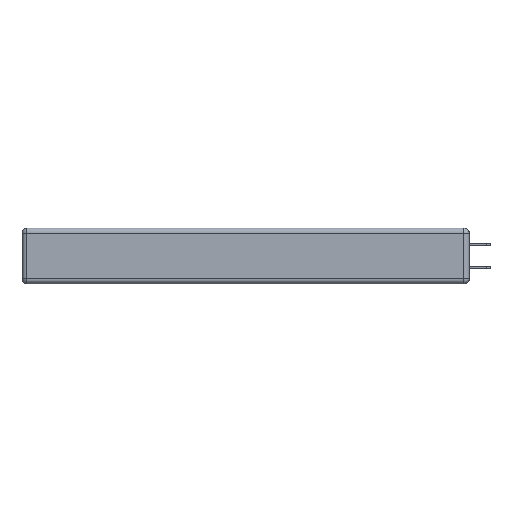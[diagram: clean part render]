
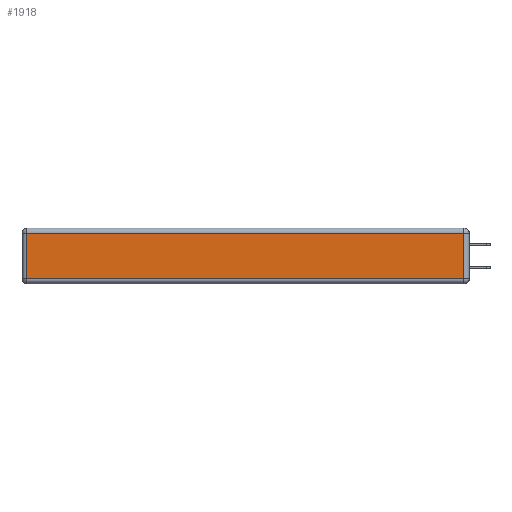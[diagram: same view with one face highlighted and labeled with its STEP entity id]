
A CAD part, left-side view. The second image highlights one B-rep face of the part: STEP entity #1918.
In plain terms, the highlighted planar face has unit normal (-1, 0, 0).
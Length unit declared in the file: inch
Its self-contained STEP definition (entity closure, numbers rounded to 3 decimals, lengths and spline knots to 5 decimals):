
#1327 = VECTOR ( 'NONE', #1982, 39.37008 ) ;
#1918 = ADVANCED_FACE ( 'NONE', ( #12549 ), #13096, .T. ) ;
#1982 = DIRECTION ( 'NONE',  ( 0., 1., 0. ) ) ;
#2371 = LINE ( 'NONE', #9660, #13173 ) ;
#2747 = ORIENTED_EDGE ( 'NONE', *, *, #12904, .T. ) ;
#2912 = AXIS2_PLACEMENT_3D ( 'NONE', #13278, #8189, #12278 ) ;
#3001 = ORIENTED_EDGE ( 'NONE', *, *, #13464, .T. ) ;
#4315 = VERTEX_POINT ( 'NONE', #12604 ) ;
#4664 = EDGE_CURVE ( 'NONE', #5330, #4315, #2371, .T. ) ;
#4808 = LINE ( 'NONE', #6531, #10383 ) ;
#5114 = CARTESIAN_POINT ( 'NONE',  ( 0., 2.72, -0.03 ) ) ;
#5116 = LINE ( 'NONE', #10831, #12792 ) ;
#5330 = VERTEX_POINT ( 'NONE', #13108 ) ;
#6531 = CARTESIAN_POINT ( 'NONE',  ( 0., 0., -0.313 ) ) ;
#7487 = EDGE_CURVE ( 'NONE', #4315, #8409, #12140, .T. ) ;
#8148 = CARTESIAN_POINT ( 'NONE',  ( 0., 2.72, -0.313 ) ) ;
#8189 = DIRECTION ( 'NONE',  ( -1., 0., 0. ) ) ;
#8409 = VERTEX_POINT ( 'NONE', #5114 ) ;
#9660 = CARTESIAN_POINT ( 'NONE',  ( 0., 0.03, -0.343 ) ) ;
#9910 = ORIENTED_EDGE ( 'NONE', *, *, #7487, .T. ) ;
#9973 = ORIENTED_EDGE ( 'NONE', *, *, #4664, .T. ) ;
#10188 = VERTEX_POINT ( 'NONE', #8148 ) ;
#10383 = VECTOR ( 'NONE', #12887, 39.37008 ) ;
#10702 = DIRECTION ( 'NONE',  ( 0., 0., -1. ) ) ;
#10831 = CARTESIAN_POINT ( 'NONE',  ( 0., 2.72, -0.343 ) ) ;
#10891 = EDGE_LOOP ( 'NONE', ( #2747, #9973, #9910, #3001 ) ) ;
#11318 = CARTESIAN_POINT ( 'NONE',  ( 0., 2.75, -0.03 ) ) ;
#12140 = LINE ( 'NONE', #11318, #1327 ) ;
#12278 = DIRECTION ( 'NONE',  ( 0., 0., 1. ) ) ;
#12549 = FACE_OUTER_BOUND ( 'NONE', #10891, .T. ) ;
#12604 = CARTESIAN_POINT ( 'NONE',  ( 0., 0.03, -0.03 ) ) ;
#12772 = DIRECTION ( 'NONE',  ( 0., 0., 1. ) ) ;
#12792 = VECTOR ( 'NONE', #10702, 39.37008 ) ;
#12887 = DIRECTION ( 'NONE',  ( 0., -1., 0. ) ) ;
#12904 = EDGE_CURVE ( 'NONE', #10188, #5330, #4808, .T. ) ;
#13096 = PLANE ( 'NONE',  #2912 ) ;
#13108 = CARTESIAN_POINT ( 'NONE',  ( 0., 0.03, -0.313 ) ) ;
#13173 = VECTOR ( 'NONE', #12772, 39.37008 ) ;
#13278 = CARTESIAN_POINT ( 'NONE',  ( 0., 0., -0.343 ) ) ;
#13464 = EDGE_CURVE ( 'NONE', #8409, #10188, #5116, .T. ) ;
